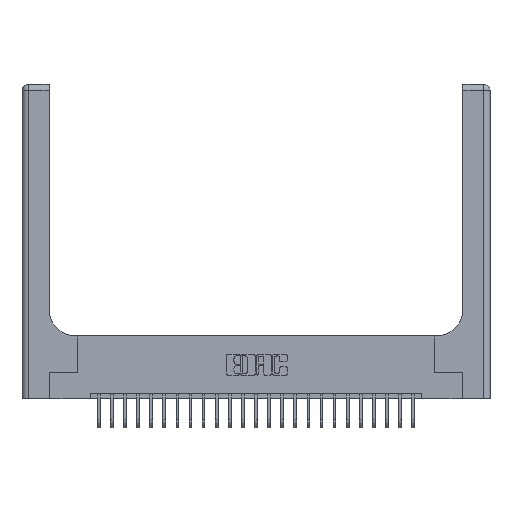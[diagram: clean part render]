
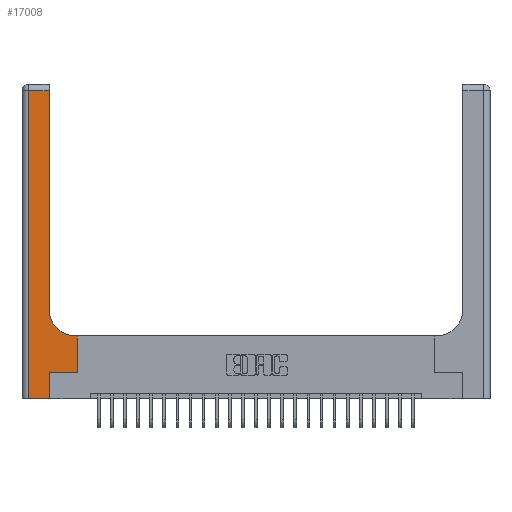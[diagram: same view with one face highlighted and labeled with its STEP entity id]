
A CAD part, top view. The second image highlights one B-rep face of the part: STEP entity #17008.
In plain terms, the highlighted planar face has unit normal (0, 0, 1).
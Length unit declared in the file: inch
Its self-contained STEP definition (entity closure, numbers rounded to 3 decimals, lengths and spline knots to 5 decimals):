
#132 = EDGE_CURVE ( 'NONE', #1681, #14348, #20212, .T. ) ;
#383 = DIRECTION ( 'NONE',  ( 0., 0., -1. ) ) ;
#1136 = ORIENTED_EDGE ( 'NONE', *, *, #13742, .T. ) ;
#1281 = CARTESIAN_POINT ( 'NONE',  ( 0.528, 0.6, 0.37 ) ) ;
#1681 = VERTEX_POINT ( 'NONE', #12557 ) ;
#1735 = VECTOR ( 'NONE', #19125, 39.37008 ) ;
#2054 = CARTESIAN_POINT ( 'NONE',  ( 0.265, 0., 0.37 ) ) ;
#4069 = AXIS2_PLACEMENT_3D ( 'NONE', #11337, #13697, #17526 ) ;
#4259 = CARTESIAN_POINT ( 'NONE',  ( 0., 0., 0.37 ) ) ;
#4371 = CARTESIAN_POINT ( 'NONE',  ( 0.265, 0., 0.37 ) ) ;
#4379 = DIRECTION ( 'NONE',  ( -1., 0., 0. ) ) ;
#4500 = DIRECTION ( 'NONE',  ( 0., 1., 0. ) ) ;
#4698 = CARTESIAN_POINT ( 'NONE',  ( 0.26, 0.6, 0.37 ) ) ;
#5692 = VECTOR ( 'NONE', #4379, 39.37008 ) ;
#6502 = CARTESIAN_POINT ( 'NONE',  ( 0.26, 3., 0.37 ) ) ;
#7130 = EDGE_LOOP ( 'NONE', ( #25749, #9357, #23938, #12920, #24252, #12895, #1136, #23883, #8506 ) ) ;
#7700 = CARTESIAN_POINT ( 'NONE',  ( 0.51, 0.6, 0.37 ) ) ;
#7924 = VECTOR ( 'NONE', #16723, 39.37008 ) ;
#8506 = ORIENTED_EDGE ( 'NONE', *, *, #16638, .T. ) ;
#8926 = DIRECTION ( 'NONE',  ( -1., 0., 0. ) ) ;
#9041 = VERTEX_POINT ( 'NONE', #13281 ) ;
#9178 = VERTEX_POINT ( 'NONE', #19337 ) ;
#9357 = ORIENTED_EDGE ( 'NONE', *, *, #132, .T. ) ;
#10117 = CARTESIAN_POINT ( 'NONE',  ( 0.06, 3., 0.37 ) ) ;
#10396 = VECTOR ( 'NONE', #18568, 39.37008 ) ;
#10532 = LINE ( 'NONE', #4698, #10396 ) ;
#10730 = EDGE_CURVE ( 'NONE', #23301, #21025, #22323, .T. ) ;
#10911 = FACE_OUTER_BOUND ( 'NONE', #7130, .T. ) ;
#11226 = VERTEX_POINT ( 'NONE', #1281 ) ;
#11337 = CARTESIAN_POINT ( 'NONE',  ( 0.51, 0.85, 0.37 ) ) ;
#12083 = AXIS2_PLACEMENT_3D ( 'NONE', #18691, #383, #8926 ) ;
#12444 = CARTESIAN_POINT ( 'NONE',  ( 0., 2.94, 0.37 ) ) ;
#12557 = CARTESIAN_POINT ( 'NONE',  ( 0.26, 2.94, 0.37 ) ) ;
#12895 = ORIENTED_EDGE ( 'NONE', *, *, #15732, .T. ) ;
#12920 = ORIENTED_EDGE ( 'NONE', *, *, #10730, .T. ) ;
#12940 = CARTESIAN_POINT ( 'NONE',  ( 0.528, 0.25, 0.37 ) ) ;
#13281 = CARTESIAN_POINT ( 'NONE',  ( 0.26, 0.85, 0.37 ) ) ;
#13697 = DIRECTION ( 'NONE',  ( 0., 0., -1. ) ) ;
#13742 = EDGE_CURVE ( 'NONE', #19857, #11226, #20828, .T. ) ;
#13916 = VECTOR ( 'NONE', #18893, 39.37008 ) ;
#14222 = CIRCLE ( 'NONE', #4069, 0.25 ) ;
#14348 = VERTEX_POINT ( 'NONE', #16443 ) ;
#14995 = VECTOR ( 'NONE', #4500, 39.37008 ) ;
#15732 = EDGE_CURVE ( 'NONE', #9178, #19857, #18431, .T. ) ;
#16443 = CARTESIAN_POINT ( 'NONE',  ( 0.06, 2.94, 0.37 ) ) ;
#16471 = CARTESIAN_POINT ( 'NONE',  ( 0.265, 0.25, 0.37 ) ) ;
#16638 = EDGE_CURVE ( 'NONE', #20919, #9041, #14222, .T. ) ;
#16723 = DIRECTION ( 'NONE',  ( 0., -1., 0. ) ) ;
#16980 = EDGE_CURVE ( 'NONE', #11226, #20919, #10532, .T. ) ;
#17008 = ADVANCED_FACE ( 'NONE', ( #10911 ), #18945, .F. ) ;
#17526 = DIRECTION ( 'NONE',  ( 1., 0., 0. ) ) ;
#17925 = VECTOR ( 'NONE', #24489, 39.37008 ) ;
#17980 = DIRECTION ( 'NONE',  ( 1., 0., 0. ) ) ;
#18431 = LINE ( 'NONE', #16471, #17925 ) ;
#18568 = DIRECTION ( 'NONE',  ( -1., 0., 0. ) ) ;
#18691 = CARTESIAN_POINT ( 'NONE',  ( 0., 3., 0.37 ) ) ;
#18873 = CARTESIAN_POINT ( 'NONE',  ( 0.528, 0.25, 0.37 ) ) ;
#18893 = DIRECTION ( 'NONE',  ( 0., 1., 0. ) ) ;
#18945 = PLANE ( 'NONE',  #12083 ) ;
#19125 = DIRECTION ( 'NONE',  ( 0., 1., 0. ) ) ;
#19337 = CARTESIAN_POINT ( 'NONE',  ( 0.265, 0.25, 0.37 ) ) ;
#19699 = VECTOR ( 'NONE', #17980, 39.37008 ) ;
#19857 = VERTEX_POINT ( 'NONE', #18873 ) ;
#20212 = LINE ( 'NONE', #12444, #5692 ) ;
#20491 = LINE ( 'NONE', #6502, #13916 ) ;
#20663 = EDGE_CURVE ( 'NONE', #14348, #23301, #24752, .T. ) ;
#20828 = LINE ( 'NONE', #12940, #14995 ) ;
#20919 = VERTEX_POINT ( 'NONE', #7700 ) ;
#21025 = VERTEX_POINT ( 'NONE', #2054 ) ;
#22323 = LINE ( 'NONE', #4259, #19699 ) ;
#22580 = LINE ( 'NONE', #4371, #1735 ) ;
#22813 = EDGE_CURVE ( 'NONE', #9041, #1681, #20491, .T. ) ;
#23301 = VERTEX_POINT ( 'NONE', #25413 ) ;
#23883 = ORIENTED_EDGE ( 'NONE', *, *, #16980, .T. ) ;
#23938 = ORIENTED_EDGE ( 'NONE', *, *, #20663, .T. ) ;
#24252 = ORIENTED_EDGE ( 'NONE', *, *, #25823, .T. ) ;
#24489 = DIRECTION ( 'NONE',  ( 1., 0., 0. ) ) ;
#24752 = LINE ( 'NONE', #10117, #7924 ) ;
#25413 = CARTESIAN_POINT ( 'NONE',  ( 0.06, 0., 0.37 ) ) ;
#25749 = ORIENTED_EDGE ( 'NONE', *, *, #22813, .T. ) ;
#25823 = EDGE_CURVE ( 'NONE', #21025, #9178, #22580, .T. ) ;
